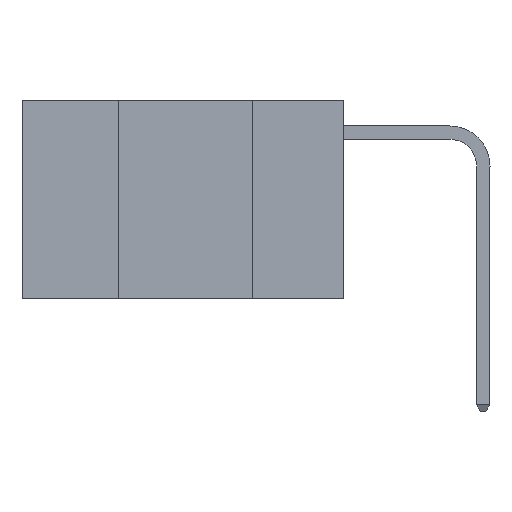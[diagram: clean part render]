
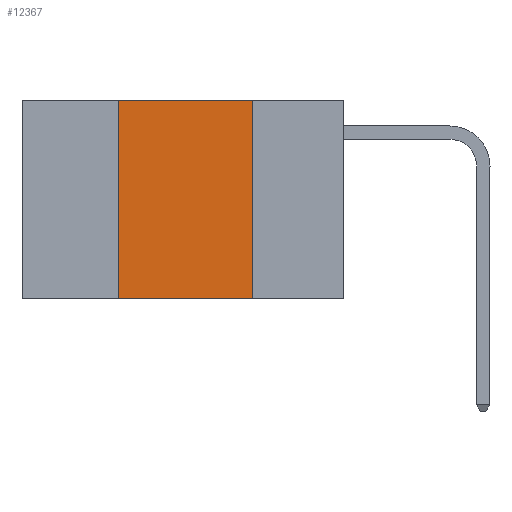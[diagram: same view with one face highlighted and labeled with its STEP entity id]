
A CAD part, left-side view. The second image highlights one B-rep face of the part: STEP entity #12367.
In plain terms, the highlighted planar face has unit normal (-1, 0, 0).
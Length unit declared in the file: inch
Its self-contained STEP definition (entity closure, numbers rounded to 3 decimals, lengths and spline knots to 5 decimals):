
#587 = CARTESIAN_POINT ( 'NONE',  ( 0., 0.6, 0. ) ) ;
#609 = EDGE_CURVE ( 'NONE', #8390, #6743, #8501, .T. ) ;
#634 = VECTOR ( 'NONE', #3767, 39.37008 ) ;
#679 = CARTESIAN_POINT ( 'NONE',  ( 0., 0.17, -0.37 ) ) ;
#768 = CARTESIAN_POINT ( 'NONE',  ( 0., 0.42, -0.37 ) ) ;
#1328 = FACE_OUTER_BOUND ( 'NONE', #9967, .T. ) ;
#1603 = AXIS2_PLACEMENT_3D ( 'NONE', #12085, #9970, #3327 ) ;
#2613 = CARTESIAN_POINT ( 'NONE',  ( 0., 0.17, 0. ) ) ;
#2775 = ORIENTED_EDGE ( 'NONE', *, *, #609, .F. ) ;
#3140 = ORIENTED_EDGE ( 'NONE', *, *, #4489, .T. ) ;
#3327 = DIRECTION ( 'NONE',  ( 0., 0., -1. ) ) ;
#3477 = VECTOR ( 'NONE', #3809, 39.37008 ) ;
#3767 = DIRECTION ( 'NONE',  ( 0., 0., -1. ) ) ;
#3809 = DIRECTION ( 'NONE',  ( 0., -1., 0. ) ) ;
#3841 = LINE ( 'NONE', #11466, #9406 ) ;
#4204 = VERTEX_POINT ( 'NONE', #768 ) ;
#4457 = EDGE_CURVE ( 'NONE', #6743, #11662, #6826, .T. ) ;
#4462 = EDGE_CURVE ( 'NONE', #4204, #8390, #3841, .T. ) ;
#4489 = EDGE_CURVE ( 'NONE', #4204, #11662, #6146, .T. ) ;
#5531 = VECTOR ( 'NONE', #11773, 39.37008 ) ;
#6146 = LINE ( 'NONE', #13659, #3477 ) ;
#6743 = VERTEX_POINT ( 'NONE', #9250 ) ;
#6826 = LINE ( 'NONE', #2613, #634 ) ;
#8390 = VERTEX_POINT ( 'NONE', #9353 ) ;
#8410 = ORIENTED_EDGE ( 'NONE', *, *, #4457, .F. ) ;
#8501 = LINE ( 'NONE', #587, #5531 ) ;
#9250 = CARTESIAN_POINT ( 'NONE',  ( 0., 0.17, 0. ) ) ;
#9353 = CARTESIAN_POINT ( 'NONE',  ( 0., 0.42, 0. ) ) ;
#9406 = VECTOR ( 'NONE', #12547, 39.37008 ) ;
#9967 = EDGE_LOOP ( 'NONE', ( #8410, #2775, #11602, #3140 ) ) ;
#9970 = DIRECTION ( 'NONE',  ( 1., 0., 0. ) ) ;
#11466 = CARTESIAN_POINT ( 'NONE',  ( 0., 0.42, 0. ) ) ;
#11602 = ORIENTED_EDGE ( 'NONE', *, *, #4462, .F. ) ;
#11662 = VERTEX_POINT ( 'NONE', #679 ) ;
#11773 = DIRECTION ( 'NONE',  ( 0., -1., 0. ) ) ;
#12085 = CARTESIAN_POINT ( 'NONE',  ( 0., 0.6, 0. ) ) ;
#12367 = ADVANCED_FACE ( 'NONE', ( #1328 ), #14207, .F. ) ;
#12547 = DIRECTION ( 'NONE',  ( 0., 0., 1. ) ) ;
#13659 = CARTESIAN_POINT ( 'NONE',  ( 0., 0.6, -0.37 ) ) ;
#14207 = PLANE ( 'NONE',  #1603 ) ;
